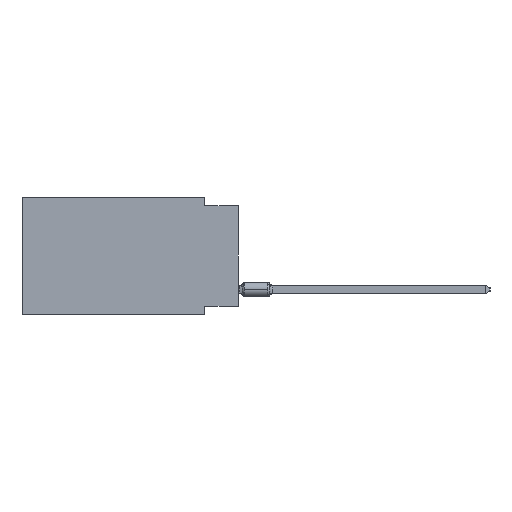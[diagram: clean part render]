
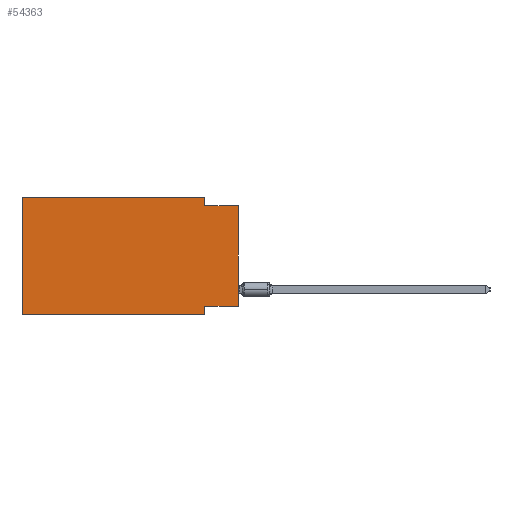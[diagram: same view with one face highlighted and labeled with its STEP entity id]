
A CAD part, left-side view. The second image highlights one B-rep face of the part: STEP entity #54363.
In plain terms, the highlighted planar face has unit normal (-1, 0, 0).
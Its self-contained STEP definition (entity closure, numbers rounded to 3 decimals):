
#488 = VERTEX_POINT ( 'NONE', #29854 ) ;
#915 = CARTESIAN_POINT ( 'NONE',  ( 0., 0., -8.255 ) ) ;
#1447 = VERTEX_POINT ( 'NONE', #57908 ) ;
#1717 = EDGE_CURVE ( 'NONE', #26610, #18641, #36614, .T. ) ;
#2381 = ORIENTED_EDGE ( 'NONE', *, *, #35881, .T. ) ;
#3305 = CARTESIAN_POINT ( 'NONE',  ( 0., 2.54, -8.89 ) ) ;
#5084 = VECTOR ( 'NONE', #32805, 1000. ) ;
#5695 = VECTOR ( 'NONE', #17495, 1000. ) ;
#7120 = LINE ( 'NONE', #38627, #25521 ) ;
#7348 = EDGE_CURVE ( 'NONE', #488, #47387, #12907, .T. ) ;
#7779 = LINE ( 'NONE', #3305, #10529 ) ;
#9149 = CARTESIAN_POINT ( 'NONE',  ( 0., 2.54, -8.89 ) ) ;
#9736 = EDGE_CURVE ( 'NONE', #39669, #27165, #7779, .T. ) ;
#10089 = EDGE_CURVE ( 'NONE', #18641, #1447, #13339, .T. ) ;
#10167 = DIRECTION ( 'NONE',  ( 0., 0., -1. ) ) ;
#10209 = LINE ( 'NONE', #41713, #5084 ) ;
#10529 = VECTOR ( 'NONE', #22042, 1000. ) ;
#10660 = CARTESIAN_POINT ( 'NONE',  ( 0., 16.383, -8.89 ) ) ;
#12907 = LINE ( 'NONE', #39680, #42641 ) ;
#13296 = ORIENTED_EDGE ( 'NONE', *, *, #1717, .F. ) ;
#13339 = LINE ( 'NONE', #49582, #5695 ) ;
#13506 = EDGE_CURVE ( 'NONE', #47387, #26610, #10209, .T. ) ;
#13693 = VECTOR ( 'NONE', #14039, 1000. ) ;
#14039 = DIRECTION ( 'NONE',  ( 0., 0., -1. ) ) ;
#15060 = ORIENTED_EDGE ( 'NONE', *, *, #17370, .F. ) ;
#15240 = CARTESIAN_POINT ( 'NONE',  ( 0., 16.383, 0. ) ) ;
#16856 = ORIENTED_EDGE ( 'NONE', *, *, #7348, .F. ) ;
#17370 = EDGE_CURVE ( 'NONE', #44596, #39669, #55889, .T. ) ;
#17495 = DIRECTION ( 'NONE',  ( 0., -1., 0. ) ) ;
#17987 = DIRECTION ( 'NONE',  ( 0., 0., 1. ) ) ;
#18641 = VERTEX_POINT ( 'NONE', #46950 ) ;
#19557 = EDGE_CURVE ( 'NONE', #44596, #1447, #7120, .T. ) ;
#19703 = DIRECTION ( 'NONE',  ( 1., 0., 0. ) ) ;
#20220 = DIRECTION ( 'NONE',  ( 0., 1., 0. ) ) ;
#22042 = DIRECTION ( 'NONE',  ( 0., 0., -1. ) ) ;
#25458 = CARTESIAN_POINT ( 'NONE',  ( 0., 2.54, 0. ) ) ;
#25521 = VECTOR ( 'NONE', #56769, 1000. ) ;
#26546 = VECTOR ( 'NONE', #41571, 1000. ) ;
#26610 = VERTEX_POINT ( 'NONE', #25458 ) ;
#26856 = ORIENTED_EDGE ( 'NONE', *, *, #9736, .F. ) ;
#27165 = VERTEX_POINT ( 'NONE', #9149 ) ;
#29854 = CARTESIAN_POINT ( 'NONE',  ( 0., 16.383, -8.89 ) ) ;
#31150 = AXIS2_PLACEMENT_3D ( 'NONE', #42253, #19703, #10167 ) ;
#32805 = DIRECTION ( 'NONE',  ( 0., -1., 0. ) ) ;
#35881 = EDGE_CURVE ( 'NONE', #488, #27165, #37416, .T. ) ;
#36614 = LINE ( 'NONE', #54737, #13693 ) ;
#37416 = LINE ( 'NONE', #10660, #26546 ) ;
#38627 = CARTESIAN_POINT ( 'NONE',  ( 0., 0., 0. ) ) ;
#39669 = VERTEX_POINT ( 'NONE', #54054 ) ;
#39680 = CARTESIAN_POINT ( 'NONE',  ( 0., 16.383, 0. ) ) ;
#41571 = DIRECTION ( 'NONE',  ( 0., -1., 0. ) ) ;
#41713 = CARTESIAN_POINT ( 'NONE',  ( 0., 16.383, 0. ) ) ;
#42253 = CARTESIAN_POINT ( 'NONE',  ( 0., 16.383, 0. ) ) ;
#42641 = VECTOR ( 'NONE', #17987, 1000. ) ;
#44596 = VERTEX_POINT ( 'NONE', #58773 ) ;
#46426 = PLANE ( 'NONE',  #31150 ) ;
#46950 = CARTESIAN_POINT ( 'NONE',  ( 0., 2.54, -0.635 ) ) ;
#47387 = VERTEX_POINT ( 'NONE', #15240 ) ;
#48095 = VECTOR ( 'NONE', #20220, 1000. ) ;
#49582 = CARTESIAN_POINT ( 'NONE',  ( 0., 0., -0.635 ) ) ;
#50272 = ORIENTED_EDGE ( 'NONE', *, *, #13506, .F. ) ;
#51364 = ORIENTED_EDGE ( 'NONE', *, *, #10089, .F. ) ;
#51465 = FACE_OUTER_BOUND ( 'NONE', #52013, .T. ) ;
#52013 = EDGE_LOOP ( 'NONE', ( #54182, #51364, #13296, #50272, #16856, #2381, #26856, #15060 ) ) ;
#54054 = CARTESIAN_POINT ( 'NONE',  ( 0., 2.54, -8.255 ) ) ;
#54182 = ORIENTED_EDGE ( 'NONE', *, *, #19557, .T. ) ;
#54363 = ADVANCED_FACE ( 'NONE', ( #51465 ), #46426, .F. ) ;
#54737 = CARTESIAN_POINT ( 'NONE',  ( 0., 2.54, 0. ) ) ;
#55889 = LINE ( 'NONE', #915, #48095 ) ;
#56769 = DIRECTION ( 'NONE',  ( 0., 0., 1. ) ) ;
#57908 = CARTESIAN_POINT ( 'NONE',  ( 0., 0., -0.635 ) ) ;
#58773 = CARTESIAN_POINT ( 'NONE',  ( 0., 0., -8.255 ) ) ;
